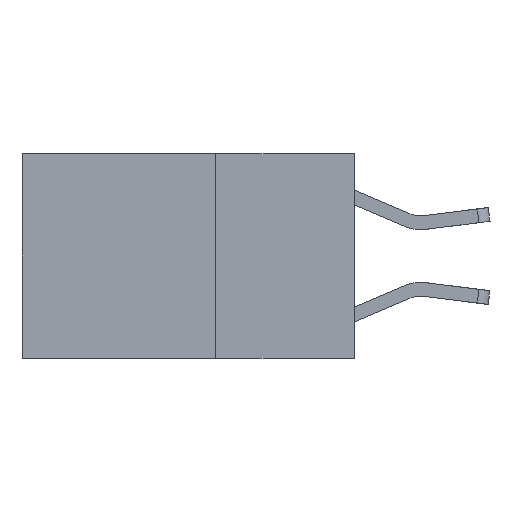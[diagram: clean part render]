
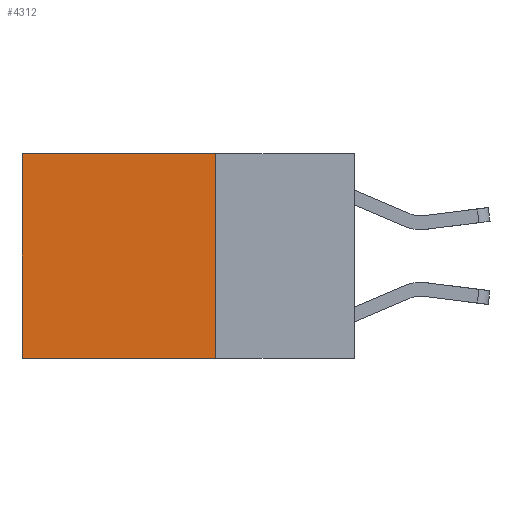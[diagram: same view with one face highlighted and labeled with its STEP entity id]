
A CAD part, left-side view. The second image highlights one B-rep face of the part: STEP entity #4312.
In plain terms, the highlighted planar face has unit normal (-1, 0, 0).
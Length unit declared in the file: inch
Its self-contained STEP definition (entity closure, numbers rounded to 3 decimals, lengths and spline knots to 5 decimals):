
#525 = PLANE ( 'NONE',  #9605 ) ;
#755 = CARTESIAN_POINT ( 'NONE',  ( 0.2625, 0.25, 0. ) ) ;
#1220 = EDGE_CURVE ( 'NONE', #6310, #9288, #6157, .T. ) ;
#1395 = VECTOR ( 'NONE', #8023, 39.37008 ) ;
#1468 = EDGE_LOOP ( 'NONE', ( #5772, #7611, #2474, #1977 ) ) ;
#1754 = DIRECTION ( 'NONE',  ( 0., 1., 0. ) ) ;
#1864 = CARTESIAN_POINT ( 'NONE',  ( 0.2625, 0.25, -0.37 ) ) ;
#1940 = DIRECTION ( 'NONE',  ( 0., 1., 0. ) ) ;
#1977 = ORIENTED_EDGE ( 'NONE', *, *, #2291, .T. ) ;
#2027 = CARTESIAN_POINT ( 'NONE',  ( 0.2625, 0.25, 0. ) ) ;
#2291 = EDGE_CURVE ( 'NONE', #6310, #2300, #8974, .T. ) ;
#2300 = VERTEX_POINT ( 'NONE', #8626 ) ;
#2474 = ORIENTED_EDGE ( 'NONE', *, *, #1220, .F. ) ;
#2902 = VERTEX_POINT ( 'NONE', #4385 ) ;
#3702 = CARTESIAN_POINT ( 'NONE',  ( 0.2625, 0.6, 0. ) ) ;
#4312 = ADVANCED_FACE ( 'NONE', ( #5603 ), #525, .F. ) ;
#4385 = CARTESIAN_POINT ( 'NONE',  ( 0.2625, 0.6, -0.37 ) ) ;
#4781 = DIRECTION ( 'NONE',  ( 0., 0., -1. ) ) ;
#4986 = VECTOR ( 'NONE', #9539, 39.37008 ) ;
#5603 = FACE_OUTER_BOUND ( 'NONE', #1468, .T. ) ;
#5772 = ORIENTED_EDGE ( 'NONE', *, *, #7629, .T. ) ;
#6157 = LINE ( 'NONE', #2027, #1395 ) ;
#6195 = CARTESIAN_POINT ( 'NONE',  ( 0.2625, 0.25, 0. ) ) ;
#6310 = VERTEX_POINT ( 'NONE', #755 ) ;
#6515 = VECTOR ( 'NONE', #1940, 39.37008 ) ;
#6943 = LINE ( 'NONE', #3702, #4986 ) ;
#7056 = EDGE_CURVE ( 'NONE', #9288, #2902, #10185, .T. ) ;
#7611 = ORIENTED_EDGE ( 'NONE', *, *, #7056, .F. ) ;
#7629 = EDGE_CURVE ( 'NONE', #2300, #2902, #6943, .T. ) ;
#8002 = VECTOR ( 'NONE', #1754, 39.37008 ) ;
#8023 = DIRECTION ( 'NONE',  ( 0., 0., -1. ) ) ;
#8094 = CARTESIAN_POINT ( 'NONE',  ( 0.2625, 0.25, 0. ) ) ;
#8626 = CARTESIAN_POINT ( 'NONE',  ( 0.2625, 0.6, 0. ) ) ;
#8974 = LINE ( 'NONE', #6195, #6515 ) ;
#9288 = VERTEX_POINT ( 'NONE', #1864 ) ;
#9539 = DIRECTION ( 'NONE',  ( 0., 0., -1. ) ) ;
#9605 = AXIS2_PLACEMENT_3D ( 'NONE', #8094, #9756, #4781 ) ;
#9756 = DIRECTION ( 'NONE',  ( 1., 0., 0. ) ) ;
#10084 = CARTESIAN_POINT ( 'NONE',  ( 0.2625, 0.25, -0.37 ) ) ;
#10185 = LINE ( 'NONE', #10084, #8002 ) ;
